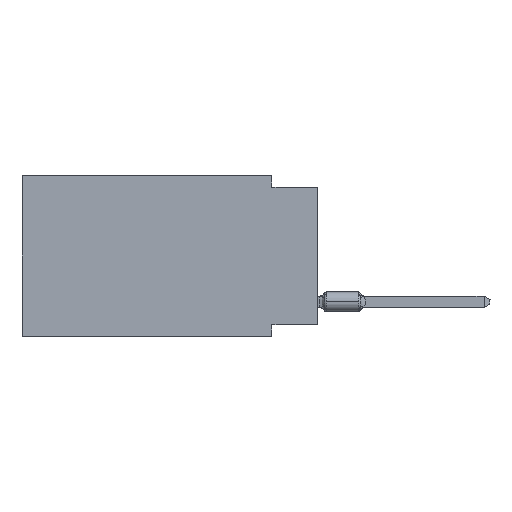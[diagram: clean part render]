
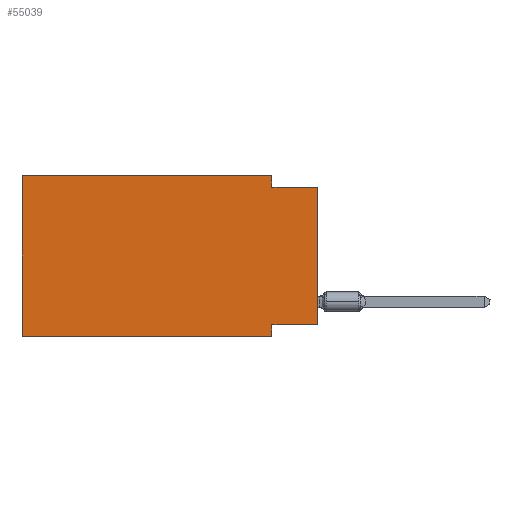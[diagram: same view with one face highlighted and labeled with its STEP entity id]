
A CAD part, left-side view. The second image highlights one B-rep face of the part: STEP entity #55039.
In plain terms, the highlighted planar face has unit normal (-1, 0, 0).
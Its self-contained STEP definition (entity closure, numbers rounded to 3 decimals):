
#470 = LINE ( 'NONE', #14571, #16105 ) ;
#474 = EDGE_CURVE ( 'NONE', #725, #53115, #6419, .T. ) ;
#595 = ORIENTED_EDGE ( 'NONE', *, *, #62537, .F. ) ;
#725 = VERTEX_POINT ( 'NONE', #60469 ) ;
#845 = CARTESIAN_POINT ( 'NONE',  ( 0., 16.383, 0. ) ) ;
#1031 = VECTOR ( 'NONE', #63079, 1000. ) ;
#3385 = EDGE_LOOP ( 'NONE', ( #63776, #13272, #595, #36085, #59956, #21836, #28997, #20278 ) ) ;
#3501 = DIRECTION ( 'NONE',  ( 0., 0., 1. ) ) ;
#4115 = DIRECTION ( 'NONE',  ( 0., 0., -1. ) ) ;
#4697 = DIRECTION ( 'NONE',  ( 0., 0., -1. ) ) ;
#5188 = VECTOR ( 'NONE', #3501, 1000. ) ;
#5713 = DIRECTION ( 'NONE',  ( 0., 0., -1. ) ) ;
#6419 = LINE ( 'NONE', #845, #7236 ) ;
#7236 = VECTOR ( 'NONE', #61166, 1000. ) ;
#8394 = EDGE_CURVE ( 'NONE', #51926, #35673, #470, .T. ) ;
#9860 = DIRECTION ( 'NONE',  ( 0., -1., 0. ) ) ;
#9898 = CARTESIAN_POINT ( 'NONE',  ( 0., 2.54, -8.89 ) ) ;
#9922 = EDGE_CURVE ( 'NONE', #62622, #35673, #33520, .T. ) ;
#10896 = CARTESIAN_POINT ( 'NONE',  ( 0., 0., 0. ) ) ;
#12568 = EDGE_CURVE ( 'NONE', #62622, #725, #53636, .T. ) ;
#12860 = EDGE_CURVE ( 'NONE', #36168, #51926, #28330, .T. ) ;
#13272 = ORIENTED_EDGE ( 'NONE', *, *, #55737, .F. ) ;
#14515 = CARTESIAN_POINT ( 'NONE',  ( 0., 2.54, 0. ) ) ;
#14571 = CARTESIAN_POINT ( 'NONE',  ( 0., 2.54, -8.89 ) ) ;
#16105 = VECTOR ( 'NONE', #5713, 1000. ) ;
#17815 = CARTESIAN_POINT ( 'NONE',  ( 0., 16.383, -8.89 ) ) ;
#18021 = VERTEX_POINT ( 'NONE', #60385 ) ;
#20278 = ORIENTED_EDGE ( 'NONE', *, *, #12860, .F. ) ;
#20713 = DIRECTION ( 'NONE',  ( 0., 0., 1. ) ) ;
#21227 = EDGE_CURVE ( 'NONE', #36168, #18021, #59714, .T. ) ;
#21733 = CARTESIAN_POINT ( 'NONE',  ( 0., 2.54, 0. ) ) ;
#21836 = ORIENTED_EDGE ( 'NONE', *, *, #9922, .T. ) ;
#22522 = VECTOR ( 'NONE', #48273, 1000. ) ;
#28330 = LINE ( 'NONE', #42756, #1031 ) ;
#28997 = ORIENTED_EDGE ( 'NONE', *, *, #8394, .F. ) ;
#31633 = VECTOR ( 'NONE', #20713, 1000. ) ;
#32526 = VERTEX_POINT ( 'NONE', #37769 ) ;
#33520 = LINE ( 'NONE', #17815, #22522 ) ;
#34752 = LINE ( 'NONE', #54753, #61564 ) ;
#35463 = CARTESIAN_POINT ( 'NONE',  ( 0., 2.54, -8.255 ) ) ;
#35673 = VERTEX_POINT ( 'NONE', #9898 ) ;
#36085 = ORIENTED_EDGE ( 'NONE', *, *, #474, .F. ) ;
#36168 = VERTEX_POINT ( 'NONE', #39938 ) ;
#37769 = CARTESIAN_POINT ( 'NONE',  ( 0., 2.54, -0.635 ) ) ;
#39938 = CARTESIAN_POINT ( 'NONE',  ( 0., 0., -8.255 ) ) ;
#42756 = CARTESIAN_POINT ( 'NONE',  ( 0., 0., -8.255 ) ) ;
#43380 = LINE ( 'NONE', #14515, #62035 ) ;
#47146 = CARTESIAN_POINT ( 'NONE',  ( 0., 16.383, -8.89 ) ) ;
#48273 = DIRECTION ( 'NONE',  ( 0., -1., 0. ) ) ;
#48319 = AXIS2_PLACEMENT_3D ( 'NONE', #59188, #64095, #4115 ) ;
#51926 = VERTEX_POINT ( 'NONE', #35463 ) ;
#53115 = VERTEX_POINT ( 'NONE', #21733 ) ;
#53619 = PLANE ( 'NONE',  #48319 ) ;
#53636 = LINE ( 'NONE', #58533, #5188 ) ;
#54753 = CARTESIAN_POINT ( 'NONE',  ( 0., 0., -0.635 ) ) ;
#55039 = ADVANCED_FACE ( 'NONE', ( #63759 ), #53619, .F. ) ;
#55737 = EDGE_CURVE ( 'NONE', #32526, #18021, #34752, .T. ) ;
#58533 = CARTESIAN_POINT ( 'NONE',  ( 0., 16.383, 0. ) ) ;
#59188 = CARTESIAN_POINT ( 'NONE',  ( 0., 16.383, 0. ) ) ;
#59714 = LINE ( 'NONE', #10896, #31633 ) ;
#59956 = ORIENTED_EDGE ( 'NONE', *, *, #12568, .F. ) ;
#60385 = CARTESIAN_POINT ( 'NONE',  ( 0., 0., -0.635 ) ) ;
#60469 = CARTESIAN_POINT ( 'NONE',  ( 0., 16.383, 0. ) ) ;
#61166 = DIRECTION ( 'NONE',  ( 0., -1., 0. ) ) ;
#61564 = VECTOR ( 'NONE', #9860, 1000. ) ;
#62035 = VECTOR ( 'NONE', #4697, 1000. ) ;
#62537 = EDGE_CURVE ( 'NONE', #53115, #32526, #43380, .T. ) ;
#62622 = VERTEX_POINT ( 'NONE', #47146 ) ;
#63079 = DIRECTION ( 'NONE',  ( 0., 1., 0. ) ) ;
#63759 = FACE_OUTER_BOUND ( 'NONE', #3385, .T. ) ;
#63776 = ORIENTED_EDGE ( 'NONE', *, *, #21227, .T. ) ;
#64095 = DIRECTION ( 'NONE',  ( 1., 0., 0. ) ) ;
